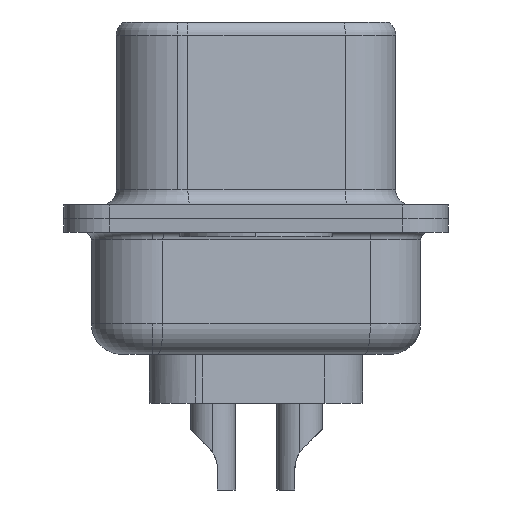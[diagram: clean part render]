
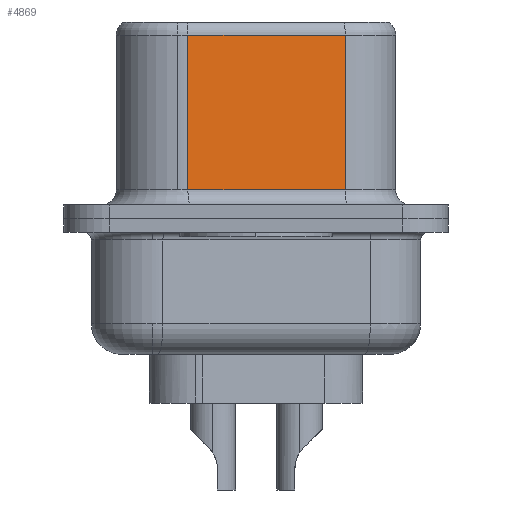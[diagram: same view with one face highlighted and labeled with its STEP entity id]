
A CAD part, left-side view. The second image highlights one B-rep face of the part: STEP entity #4869.
In plain terms, the highlighted planar face has unit normal (-0.985, -0.174, 0).
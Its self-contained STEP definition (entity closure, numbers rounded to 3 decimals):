
#62 = ORIENTED_EDGE ( 'NONE', *, *, #3856, .F. ) ;
#283 = LINE ( 'NONE', #19627, #11003 ) ;
#430 = ORIENTED_EDGE ( 'NONE', *, *, #6780, .T. ) ;
#1158 = VERTEX_POINT ( 'NONE', #18242 ) ;
#1393 = ORIENTED_EDGE ( 'NONE', *, *, #7005, .T. ) ;
#1862 = DIRECTION ( 'NONE',  ( -0.174, 0.985, 0. ) ) ;
#2416 = CARTESIAN_POINT ( 'NONE',  ( 4.58, -2.927, 6.52 ) ) ;
#2447 = VECTOR ( 'NONE', #3785, 1000. ) ;
#3219 = EDGE_LOOP ( 'NONE', ( #62, #1393, #430, #8307 ) ) ;
#3785 = DIRECTION ( 'NONE',  ( 0., 0., -1. ) ) ;
#3856 = EDGE_CURVE ( 'NONE', #9637, #4628, #18279, .T. ) ;
#4335 = CARTESIAN_POINT ( 'NONE',  ( 4.58, -2.927, 6.52 ) ) ;
#4628 = VERTEX_POINT ( 'NONE', #16596 ) ;
#4869 = ADVANCED_FACE ( 'NONE', ( #12355 ), #7522, .F. ) ;
#6780 = EDGE_CURVE ( 'NONE', #1158, #16616, #20783, .T. ) ;
#7005 = EDGE_CURVE ( 'NONE', #9637, #1158, #9914, .T. ) ;
#7007 = EDGE_CURVE ( 'NONE', #16616, #4628, #283, .T. ) ;
#7522 = PLANE ( 'NONE',  #17110 ) ;
#8307 = ORIENTED_EDGE ( 'NONE', *, *, #7007, .T. ) ;
#8902 = DIRECTION ( 'NONE',  ( -0.174, 0.985, 0. ) ) ;
#9637 = VERTEX_POINT ( 'NONE', #10349 ) ;
#9914 = LINE ( 'NONE', #16345, #10006 ) ;
#10006 = VECTOR ( 'NONE', #1862, 1000. ) ;
#10349 = CARTESIAN_POINT ( 'NONE',  ( 4.58, -2.927, 6.02 ) ) ;
#11003 = VECTOR ( 'NONE', #11586, 1000. ) ;
#11586 = DIRECTION ( 'NONE',  ( 0.174, -0.985, 0. ) ) ;
#12355 = FACE_OUTER_BOUND ( 'NONE', #3219, .T. ) ;
#15510 = VECTOR ( 'NONE', #19319, 1000. ) ;
#16345 = CARTESIAN_POINT ( 'NONE',  ( 4.58, -2.927, 6.02 ) ) ;
#16557 = CARTESIAN_POINT ( 'NONE',  ( 3.67, 2.233, 0.95 ) ) ;
#16596 = CARTESIAN_POINT ( 'NONE',  ( 4.58, -2.927, 0.95 ) ) ;
#16616 = VERTEX_POINT ( 'NONE', #16557 ) ;
#17110 = AXIS2_PLACEMENT_3D ( 'NONE', #4335, #20087, #8902 ) ;
#18242 = CARTESIAN_POINT ( 'NONE',  ( 3.67, 2.233, 6.02 ) ) ;
#18279 = LINE ( 'NONE', #2416, #2447 ) ;
#19319 = DIRECTION ( 'NONE',  ( 0., 0., -1. ) ) ;
#19627 = CARTESIAN_POINT ( 'NONE',  ( 4.58, -2.927, 0.95 ) ) ;
#20087 = DIRECTION ( 'NONE',  ( 0.985, 0.174, 0. ) ) ;
#20783 = LINE ( 'NONE', #20885, #15510 ) ;
#20885 = CARTESIAN_POINT ( 'NONE',  ( 3.67, 2.233, 6.52 ) ) ;
